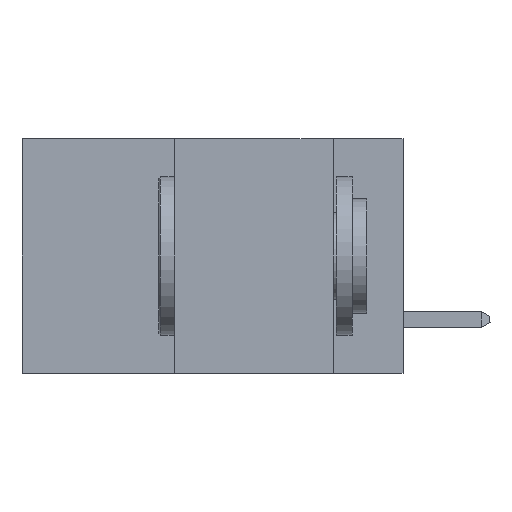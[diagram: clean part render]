
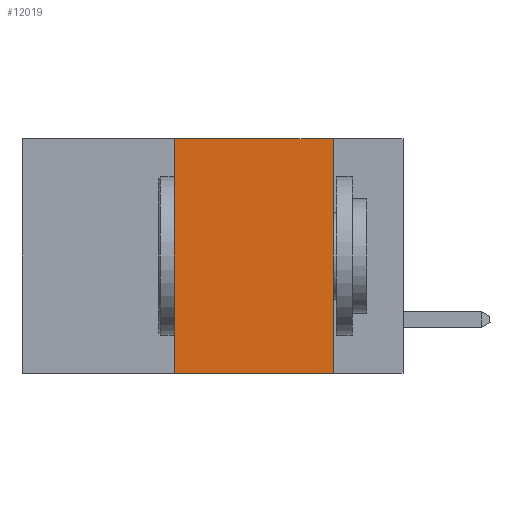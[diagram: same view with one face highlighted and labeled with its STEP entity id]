
A CAD part, left-side view. The second image highlights one B-rep face of the part: STEP entity #12019.
In plain terms, the highlighted planar face has unit normal (-1, 0, 0).
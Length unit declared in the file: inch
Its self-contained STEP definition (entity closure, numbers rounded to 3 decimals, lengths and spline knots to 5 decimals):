
#99 = AXIS2_PLACEMENT_3D ( 'NONE', #10608, #1370, #4449 ) ;
#768 = CARTESIAN_POINT ( 'NONE',  ( 0., 0.36, 0. ) ) ;
#1172 = VERTEX_POINT ( 'NONE', #768 ) ;
#1316 = DIRECTION ( 'NONE',  ( 0., -1., 0. ) ) ;
#1335 = ORIENTED_EDGE ( 'NONE', *, *, #9950, .F. ) ;
#1370 = DIRECTION ( 'NONE',  ( 1., 0., 0. ) ) ;
#1623 = VERTEX_POINT ( 'NONE', #6056 ) ;
#1705 = CARTESIAN_POINT ( 'NONE',  ( 0., 0.36, -0.37 ) ) ;
#2247 = CARTESIAN_POINT ( 'NONE',  ( 0., 0.11, 0. ) ) ;
#3071 = DIRECTION ( 'NONE',  ( 0., 0., 1. ) ) ;
#4377 = EDGE_LOOP ( 'NONE', ( #1335, #10815, #13187, #7558 ) ) ;
#4449 = DIRECTION ( 'NONE',  ( 0., 0., -1. ) ) ;
#4537 = LINE ( 'NONE', #12402, #5519 ) ;
#4956 = CARTESIAN_POINT ( 'NONE',  ( 0., 0.11, 0. ) ) ;
#5468 = LINE ( 'NONE', #6486, #9911 ) ;
#5519 = VECTOR ( 'NONE', #3071, 39.37008 ) ;
#5796 = LINE ( 'NONE', #4956, #10545 ) ;
#5959 = DIRECTION ( 'NONE',  ( 0., 0., -1. ) ) ;
#6056 = CARTESIAN_POINT ( 'NONE',  ( 0., 0.11, -0.37 ) ) ;
#6486 = CARTESIAN_POINT ( 'NONE',  ( 0., 0.6, -0.37 ) ) ;
#6490 = PLANE ( 'NONE',  #99 ) ;
#7558 = ORIENTED_EDGE ( 'NONE', *, *, #10066, .T. ) ;
#7674 = CARTESIAN_POINT ( 'NONE',  ( 0., 0.6, 0. ) ) ;
#8497 = EDGE_CURVE ( 'NONE', #8987, #1172, #4537, .T. ) ;
#8762 = VERTEX_POINT ( 'NONE', #2247 ) ;
#8783 = VECTOR ( 'NONE', #11773, 39.37008 ) ;
#8987 = VERTEX_POINT ( 'NONE', #1705 ) ;
#9254 = LINE ( 'NONE', #7674, #8783 ) ;
#9911 = VECTOR ( 'NONE', #1316, 39.37008 ) ;
#9950 = EDGE_CURVE ( 'NONE', #8762, #1623, #5796, .T. ) ;
#10066 = EDGE_CURVE ( 'NONE', #8987, #1623, #5468, .T. ) ;
#10166 = FACE_OUTER_BOUND ( 'NONE', #4377, .T. ) ;
#10254 = EDGE_CURVE ( 'NONE', #1172, #8762, #9254, .T. ) ;
#10545 = VECTOR ( 'NONE', #5959, 39.37008 ) ;
#10608 = CARTESIAN_POINT ( 'NONE',  ( 0., 0.6, 0. ) ) ;
#10815 = ORIENTED_EDGE ( 'NONE', *, *, #10254, .F. ) ;
#11773 = DIRECTION ( 'NONE',  ( 0., -1., 0. ) ) ;
#12019 = ADVANCED_FACE ( 'NONE', ( #10166 ), #6490, .F. ) ;
#12402 = CARTESIAN_POINT ( 'NONE',  ( 0., 0.36, 0. ) ) ;
#13187 = ORIENTED_EDGE ( 'NONE', *, *, #8497, .F. ) ;
